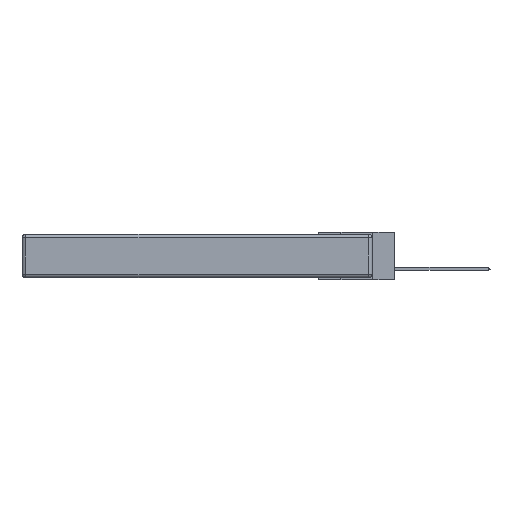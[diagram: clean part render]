
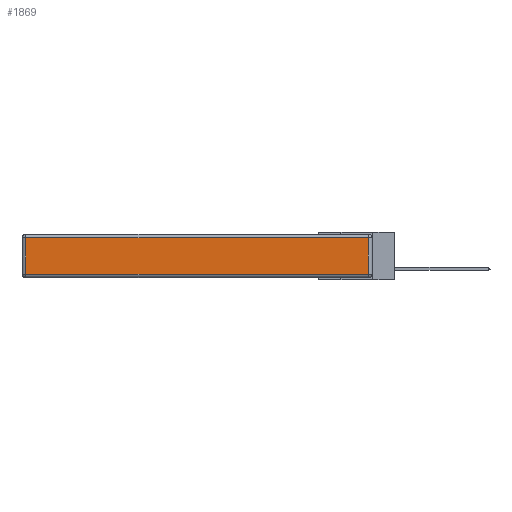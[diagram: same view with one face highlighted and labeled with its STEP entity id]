
A CAD part, left-side view. The second image highlights one B-rep face of the part: STEP entity #1869.
In plain terms, the highlighted planar face has unit normal (-1, 0, 0).
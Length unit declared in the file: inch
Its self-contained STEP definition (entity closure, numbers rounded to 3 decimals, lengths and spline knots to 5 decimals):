
#653 = VERTEX_POINT ( 'NONE', #16499 ) ;
#1216 = LINE ( 'NONE', #7050, #10733 ) ;
#1869 = ADVANCED_FACE ( 'NONE', ( #10007 ), #12858, .T. ) ;
#2475 = CARTESIAN_POINT ( 'NONE',  ( 0., 0.03, -0.313 ) ) ;
#2675 = VECTOR ( 'NONE', #15794, 39.37008 ) ;
#2804 = ORIENTED_EDGE ( 'NONE', *, *, #14156, .T. ) ;
#3905 = EDGE_LOOP ( 'NONE', ( #12989, #2804, #6705, #6047 ) ) ;
#4504 = DIRECTION ( 'NONE',  ( 0., 0., -1. ) ) ;
#5630 = CARTESIAN_POINT ( 'NONE',  ( 0., 2.75, -0.03 ) ) ;
#5714 = EDGE_CURVE ( 'NONE', #13755, #653, #18561, .T. ) ;
#5884 = CARTESIAN_POINT ( 'NONE',  ( 0., 0.03, -0.03 ) ) ;
#6047 = ORIENTED_EDGE ( 'NONE', *, *, #13037, .T. ) ;
#6311 = VERTEX_POINT ( 'NONE', #2475 ) ;
#6705 = ORIENTED_EDGE ( 'NONE', *, *, #5714, .T. ) ;
#7050 = CARTESIAN_POINT ( 'NONE',  ( 0., 0.03, -0.343 ) ) ;
#9873 = DIRECTION ( 'NONE',  ( -1., 0., 0. ) ) ;
#10007 = FACE_OUTER_BOUND ( 'NONE', #3905, .T. ) ;
#10733 = VECTOR ( 'NONE', #11337, 39.37008 ) ;
#11286 = CARTESIAN_POINT ( 'NONE',  ( 0., 2.72, -0.313 ) ) ;
#11337 = DIRECTION ( 'NONE',  ( 0., 0., 1. ) ) ;
#11473 = DIRECTION ( 'NONE',  ( 0., 0., 1. ) ) ;
#12080 = CARTESIAN_POINT ( 'NONE',  ( 0., 0., -0.313 ) ) ;
#12585 = VECTOR ( 'NONE', #17773, 39.37008 ) ;
#12858 = PLANE ( 'NONE',  #15217 ) ;
#12989 = ORIENTED_EDGE ( 'NONE', *, *, #17249, .T. ) ;
#13037 = EDGE_CURVE ( 'NONE', #653, #17921, #17352, .T. ) ;
#13145 = CARTESIAN_POINT ( 'NONE',  ( 0., 2.72, -0.343 ) ) ;
#13755 = VERTEX_POINT ( 'NONE', #5884 ) ;
#14156 = EDGE_CURVE ( 'NONE', #6311, #13755, #1216, .T. ) ;
#14364 = CARTESIAN_POINT ( 'NONE',  ( 0., 0., -0.343 ) ) ;
#14378 = LINE ( 'NONE', #12080, #12585 ) ;
#14391 = VECTOR ( 'NONE', #4504, 39.37008 ) ;
#15217 = AXIS2_PLACEMENT_3D ( 'NONE', #14364, #9873, #11473 ) ;
#15794 = DIRECTION ( 'NONE',  ( 0., 1., 0. ) ) ;
#16499 = CARTESIAN_POINT ( 'NONE',  ( 0., 2.72, -0.03 ) ) ;
#17249 = EDGE_CURVE ( 'NONE', #17921, #6311, #14378, .T. ) ;
#17352 = LINE ( 'NONE', #13145, #14391 ) ;
#17773 = DIRECTION ( 'NONE',  ( 0., -1., 0. ) ) ;
#17921 = VERTEX_POINT ( 'NONE', #11286 ) ;
#18561 = LINE ( 'NONE', #5630, #2675 ) ;
